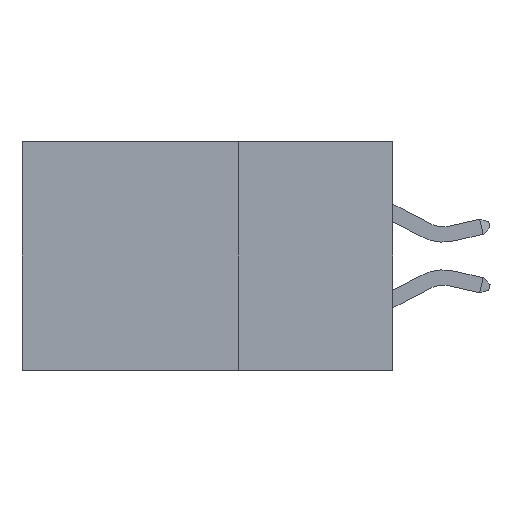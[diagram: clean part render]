
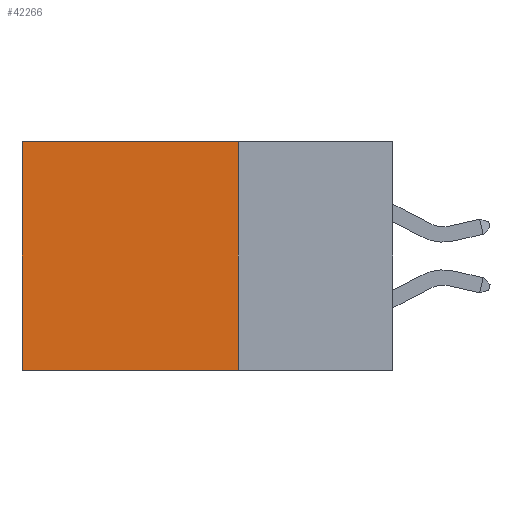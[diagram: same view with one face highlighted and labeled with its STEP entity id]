
A CAD part, left-side view. The second image highlights one B-rep face of the part: STEP entity #42266.
In plain terms, the highlighted planar face has unit normal (-1, 0, 0).
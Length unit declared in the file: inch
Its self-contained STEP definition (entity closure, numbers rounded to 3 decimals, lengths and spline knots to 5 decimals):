
#2787 = VERTEX_POINT ( 'NONE', #34309 ) ;
#2987 = LINE ( 'NONE', #6754, #38306 ) ;
#3178 = DIRECTION ( 'NONE',  ( 0., 0., -1. ) ) ;
#3650 = PLANE ( 'NONE',  #26047 ) ;
#6754 = CARTESIAN_POINT ( 'NONE',  ( 0.2875, 0.25, 0. ) ) ;
#7077 = CARTESIAN_POINT ( 'NONE',  ( 0.2875, 0.25, 0. ) ) ;
#7676 = ORIENTED_EDGE ( 'NONE', *, *, #39203, .F. ) ;
#8302 = LINE ( 'NONE', #30520, #42534 ) ;
#8387 = CARTESIAN_POINT ( 'NONE',  ( 0.2875, 0.6, -0.37 ) ) ;
#9399 = DIRECTION ( 'NONE',  ( 0., 0., -1. ) ) ;
#9622 = VECTOR ( 'NONE', #21796, 39.37008 ) ;
#12554 = FACE_OUTER_BOUND ( 'NONE', #44165, .T. ) ;
#12742 = ORIENTED_EDGE ( 'NONE', *, *, #30359, .F. ) ;
#13959 = DIRECTION ( 'NONE',  ( 0., 0., -1. ) ) ;
#16813 = LINE ( 'NONE', #19675, #24852 ) ;
#16887 = CARTESIAN_POINT ( 'NONE',  ( 0.2875, 0.25, 0. ) ) ;
#18578 = ORIENTED_EDGE ( 'NONE', *, *, #32427, .T. ) ;
#19675 = CARTESIAN_POINT ( 'NONE',  ( 0.2875, 0.6, 0. ) ) ;
#20641 = CARTESIAN_POINT ( 'NONE',  ( 0.2875, 0.25, -0.37 ) ) ;
#21796 = DIRECTION ( 'NONE',  ( 0., 1., 0. ) ) ;
#22548 = VERTEX_POINT ( 'NONE', #16887 ) ;
#24852 = VECTOR ( 'NONE', #9399, 39.37008 ) ;
#26047 = AXIS2_PLACEMENT_3D ( 'NONE', #7077, #34428, #13959 ) ;
#27251 = DIRECTION ( 'NONE',  ( 0., 1., 0. ) ) ;
#27826 = LINE ( 'NONE', #28550, #9622 ) ;
#28550 = CARTESIAN_POINT ( 'NONE',  ( 0.2875, 0.25, -0.37 ) ) ;
#30359 = EDGE_CURVE ( 'NONE', #22548, #30451, #8302, .T. ) ;
#30451 = VERTEX_POINT ( 'NONE', #20641 ) ;
#30520 = CARTESIAN_POINT ( 'NONE',  ( 0.2875, 0.25, 0. ) ) ;
#32427 = EDGE_CURVE ( 'NONE', #22548, #2787, #2987, .T. ) ;
#33404 = EDGE_CURVE ( 'NONE', #2787, #36429, #16813, .T. ) ;
#34309 = CARTESIAN_POINT ( 'NONE',  ( 0.2875, 0.6, 0. ) ) ;
#34428 = DIRECTION ( 'NONE',  ( 1., 0., 0. ) ) ;
#34855 = ORIENTED_EDGE ( 'NONE', *, *, #33404, .T. ) ;
#36429 = VERTEX_POINT ( 'NONE', #8387 ) ;
#38306 = VECTOR ( 'NONE', #27251, 39.37008 ) ;
#39203 = EDGE_CURVE ( 'NONE', #30451, #36429, #27826, .T. ) ;
#42266 = ADVANCED_FACE ( 'NONE', ( #12554 ), #3650, .F. ) ;
#42534 = VECTOR ( 'NONE', #3178, 39.37008 ) ;
#44165 = EDGE_LOOP ( 'NONE', ( #34855, #7676, #12742, #18578 ) ) ;
